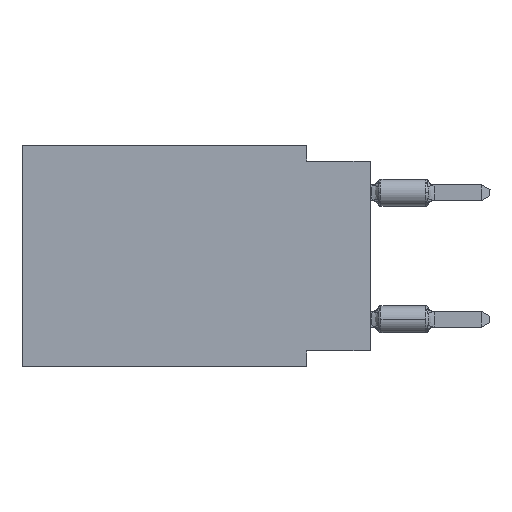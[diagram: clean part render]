
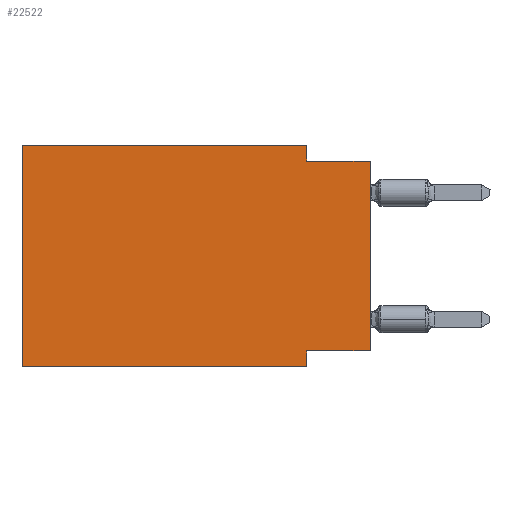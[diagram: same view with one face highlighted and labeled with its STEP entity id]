
A CAD part, left-side view. The second image highlights one B-rep face of the part: STEP entity #22522.
In plain terms, the highlighted planar face has unit normal (-1, 0, 0).
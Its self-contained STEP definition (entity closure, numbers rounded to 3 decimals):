
#130 = LINE ( 'NONE', #26780, #10566 ) ;
#2160 = EDGE_CURVE ( 'NONE', #28791, #6217, #22083, .T. ) ;
#2332 = LINE ( 'NONE', #22143, #19232 ) ;
#2480 = DIRECTION ( 'NONE',  ( 1., 0., 0. ) ) ;
#2974 = VECTOR ( 'NONE', #17379, 1000. ) ;
#3068 = EDGE_CURVE ( 'NONE', #6217, #12713, #25044, .T. ) ;
#4128 = VECTOR ( 'NONE', #18764, 1000. ) ;
#4358 = VERTEX_POINT ( 'NONE', #19693 ) ;
#4363 = CARTESIAN_POINT ( 'NONE',  ( 0., 13.97, -8.89 ) ) ;
#5272 = ORIENTED_EDGE ( 'NONE', *, *, #14304, .F. ) ;
#5502 = VECTOR ( 'NONE', #17618, 1000. ) ;
#5826 = VECTOR ( 'NONE', #22430, 1000. ) ;
#6217 = VERTEX_POINT ( 'NONE', #12300 ) ;
#7299 = VECTOR ( 'NONE', #32972, 1000. ) ;
#8427 = EDGE_CURVE ( 'NONE', #31007, #28791, #130, .T. ) ;
#8884 = ORIENTED_EDGE ( 'NONE', *, *, #3068, .F. ) ;
#9648 = CARTESIAN_POINT ( 'NONE',  ( 0., 13.97, 0. ) ) ;
#9777 = DIRECTION ( 'NONE',  ( 0., 0., 1. ) ) ;
#10566 = VECTOR ( 'NONE', #29217, 1000. ) ;
#11809 = CARTESIAN_POINT ( 'NONE',  ( 0., 0., -0.635 ) ) ;
#12235 = CARTESIAN_POINT ( 'NONE',  ( 0., 2.54, 0. ) ) ;
#12300 = CARTESIAN_POINT ( 'NONE',  ( 0., 2.54, -0.635 ) ) ;
#12327 = ORIENTED_EDGE ( 'NONE', *, *, #19871, .F. ) ;
#12551 = CARTESIAN_POINT ( 'NONE',  ( 0., 2.54, -8.255 ) ) ;
#12578 = LINE ( 'NONE', #25467, #25817 ) ;
#12713 = VERTEX_POINT ( 'NONE', #20956 ) ;
#14304 = EDGE_CURVE ( 'NONE', #25531, #19142, #14690, .T. ) ;
#14690 = LINE ( 'NONE', #25314, #7299 ) ;
#15458 = ORIENTED_EDGE ( 'NONE', *, *, #18573, .F. ) ;
#16089 = FACE_OUTER_BOUND ( 'NONE', #27166, .T. ) ;
#16259 = DIRECTION ( 'NONE',  ( 0., 0., -1. ) ) ;
#16508 = ORIENTED_EDGE ( 'NONE', *, *, #30262, .T. ) ;
#16939 = CARTESIAN_POINT ( 'NONE',  ( 0., 0., -8.255 ) ) ;
#17379 = DIRECTION ( 'NONE',  ( 0., 0., -1. ) ) ;
#17618 = DIRECTION ( 'NONE',  ( 0., -1., 0. ) ) ;
#18573 = EDGE_CURVE ( 'NONE', #4358, #31007, #18936, .T. ) ;
#18764 = DIRECTION ( 'NONE',  ( 0., 0., 1. ) ) ;
#18936 = LINE ( 'NONE', #31824, #4128 ) ;
#19142 = VERTEX_POINT ( 'NONE', #32794 ) ;
#19232 = VECTOR ( 'NONE', #26213, 1000. ) ;
#19693 = CARTESIAN_POINT ( 'NONE',  ( 0., 13.97, -8.89 ) ) ;
#19797 = ORIENTED_EDGE ( 'NONE', *, *, #2160, .F. ) ;
#19871 = EDGE_CURVE ( 'NONE', #30159, #25531, #2332, .T. ) ;
#20956 = CARTESIAN_POINT ( 'NONE',  ( 0., 0., -0.635 ) ) ;
#21649 = CARTESIAN_POINT ( 'NONE',  ( 0., 13.97, 0. ) ) ;
#22083 = LINE ( 'NONE', #33203, #2974 ) ;
#22143 = CARTESIAN_POINT ( 'NONE',  ( 0., 0., -8.255 ) ) ;
#22430 = DIRECTION ( 'NONE',  ( 0., -1., 0. ) ) ;
#22522 = ADVANCED_FACE ( 'NONE', ( #16089 ), #24261, .F. ) ;
#22992 = ORIENTED_EDGE ( 'NONE', *, *, #8427, .F. ) ;
#24261 = PLANE ( 'NONE',  #31294 ) ;
#25044 = LINE ( 'NONE', #11809, #5826 ) ;
#25314 = CARTESIAN_POINT ( 'NONE',  ( 0., 2.54, -8.89 ) ) ;
#25467 = CARTESIAN_POINT ( 'NONE',  ( 0., 0., 0. ) ) ;
#25531 = VERTEX_POINT ( 'NONE', #12551 ) ;
#25817 = VECTOR ( 'NONE', #9777, 1000. ) ;
#26213 = DIRECTION ( 'NONE',  ( 0., 1., 0. ) ) ;
#26780 = CARTESIAN_POINT ( 'NONE',  ( 0., 13.97, 0. ) ) ;
#27166 = EDGE_LOOP ( 'NONE', ( #31839, #8884, #19797, #22992, #15458, #16508, #5272, #12327 ) ) ;
#28791 = VERTEX_POINT ( 'NONE', #12235 ) ;
#29217 = DIRECTION ( 'NONE',  ( 0., -1., 0. ) ) ;
#30159 = VERTEX_POINT ( 'NONE', #16939 ) ;
#30262 = EDGE_CURVE ( 'NONE', #4358, #19142, #30839, .T. ) ;
#30839 = LINE ( 'NONE', #4363, #5502 ) ;
#31007 = VERTEX_POINT ( 'NONE', #9648 ) ;
#31294 = AXIS2_PLACEMENT_3D ( 'NONE', #21649, #2480, #16259 ) ;
#31525 = EDGE_CURVE ( 'NONE', #30159, #12713, #12578, .T. ) ;
#31824 = CARTESIAN_POINT ( 'NONE',  ( 0., 13.97, 0. ) ) ;
#31839 = ORIENTED_EDGE ( 'NONE', *, *, #31525, .T. ) ;
#32794 = CARTESIAN_POINT ( 'NONE',  ( 0., 2.54, -8.89 ) ) ;
#32972 = DIRECTION ( 'NONE',  ( 0., 0., -1. ) ) ;
#33203 = CARTESIAN_POINT ( 'NONE',  ( 0., 2.54, 0. ) ) ;
